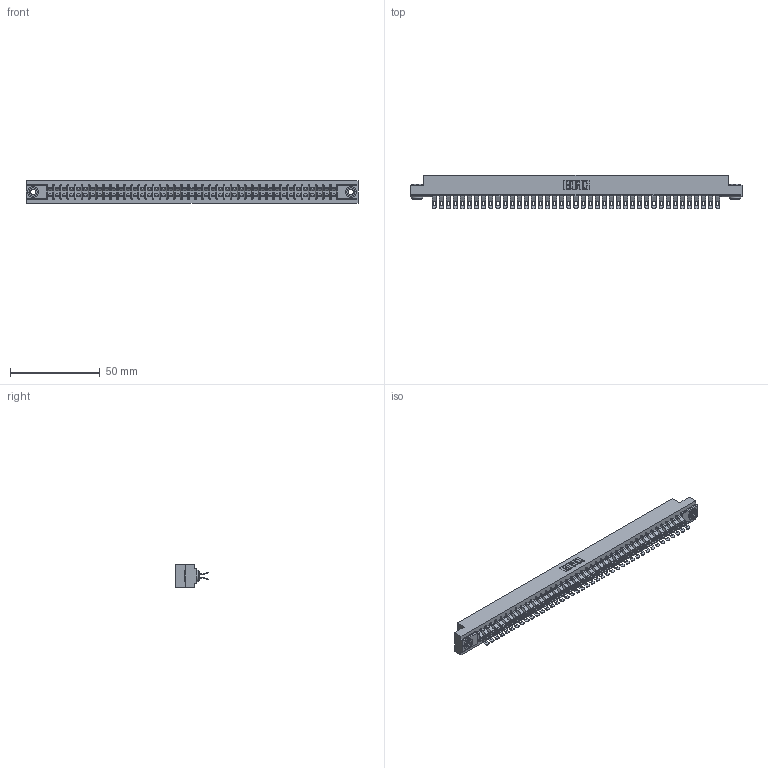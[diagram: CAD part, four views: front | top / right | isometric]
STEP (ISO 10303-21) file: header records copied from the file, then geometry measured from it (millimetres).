
FILE_DESCRIPTION (( 'STEP AP203' ), '1' );
FILE_NAME ('807-082-555-203.STEP', '2021-07-20T17:50:16', ( '' ), ( '' ), 'SwSTEP 2.0', 'SolidWorks 2020', '' );
FILE_SCHEMA (( 'CONFIG_CONTROL_DESIGN' ));
Length unit declared in the file: inch
Products named in the file (4): 307-290-001_555; 345-250-002_345-250-002-102; 807-082-555-203; 807 Part_.156 Dia Mounting Holes
Assembly tree (85 placements, depth 2):
  807-082-555-203
    807 Part_.156 Dia Mounting Holes
    307-290-001_555  x82
    345-250-002_345-250-002-102  x2
Bounding box: 185.47 x 18.75 x 12.7 mm (x, y, z)
Volume: 19961.2 mm3; surface area: 26009.9 mm2
Topology: 85 solids, 85 shells, 5214 faces, 15277 edges, 9958 vertices
Faces by surface type: plane 2882, cylinder 2240, sphere 84, cone 8
Entity records: 38186 total; most frequent: CARTESIAN_POINT 6234, ORIENTED_EDGE 6172, DIRECTION 6128, EDGE_CURVE 3086, LINE 2348, VECTOR 2348, VERTEX_POINT 1996, AXIS2_PLACEMENT_3D 1890
